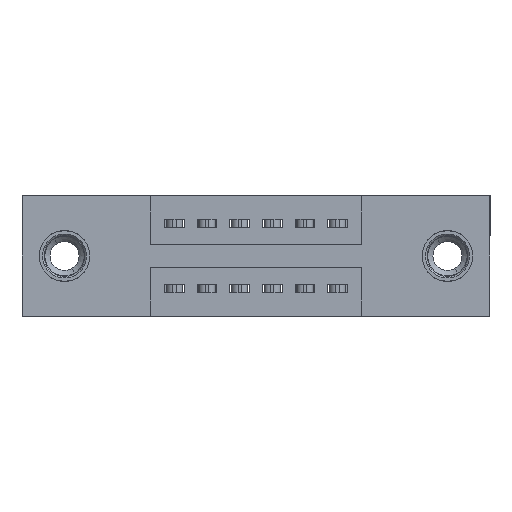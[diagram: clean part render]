
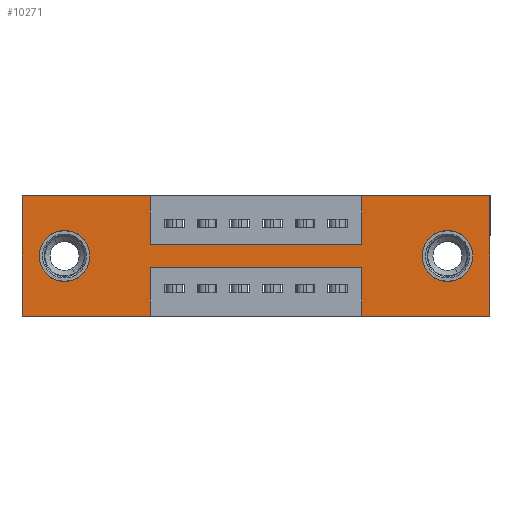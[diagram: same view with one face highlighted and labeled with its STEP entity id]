
A CAD part, front view. The second image highlights one B-rep face of the part: STEP entity #10271.
In plain terms, the highlighted planar face has unit normal (0, -1, 0).
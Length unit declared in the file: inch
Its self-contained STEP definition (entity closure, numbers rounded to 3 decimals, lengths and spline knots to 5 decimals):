
#71 = CARTESIAN_POINT ( 'NONE',  ( 1.305, 0., -0.107 ) ) ;
#195 = CARTESIAN_POINT ( 'NONE',  ( 1.0425, 0., 0. ) ) ;
#309 = FACE_BOUND ( 'NONE', #2899, .T. ) ;
#329 = VERTEX_POINT ( 'NONE', #5077 ) ;
#443 = LINE ( 'NONE', #3938, #9184 ) ;
#509 = VERTEX_POINT ( 'NONE', #8169 ) ;
#593 = VERTEX_POINT ( 'NONE', #8720 ) ;
#978 = CARTESIAN_POINT ( 'NONE',  ( 1.305, 0., -0.263 ) ) ;
#1012 = CARTESIAN_POINT ( 'NONE',  ( 1.435, 0., 0. ) ) ;
#1081 = CARTESIAN_POINT ( 'NONE',  ( 0.13, 0., -0.185 ) ) ;
#1207 = LINE ( 'NONE', #6650, #5820 ) ;
#1309 = VERTEX_POINT ( 'NONE', #8824 ) ;
#1321 = EDGE_CURVE ( 'NONE', #329, #1309, #13550, .T. ) ;
#1327 = VECTOR ( 'NONE', #13985, 39.37008 ) ;
#1766 = EDGE_CURVE ( 'NONE', #7419, #8603, #5643, .T. ) ;
#1823 = DIRECTION ( 'NONE',  ( 1., 0., 0. ) ) ;
#1833 = DIRECTION ( 'NONE',  ( -1., 0., 0. ) ) ;
#1854 = LINE ( 'NONE', #4841, #3917 ) ;
#1885 = CARTESIAN_POINT ( 'NONE',  ( 0., 0., -0.37 ) ) ;
#2115 = VECTOR ( 'NONE', #11081, 39.37008 ) ;
#2276 = VECTOR ( 'NONE', #7738, 39.37008 ) ;
#2292 = ORIENTED_EDGE ( 'NONE', *, *, #6326, .T. ) ;
#2359 = FACE_BOUND ( 'NONE', #3261, .T. ) ;
#2613 = CARTESIAN_POINT ( 'NONE',  ( 0., 0., -0.37 ) ) ;
#2625 = LINE ( 'NONE', #5478, #2115 ) ;
#2825 = ORIENTED_EDGE ( 'NONE', *, *, #12207, .F. ) ;
#2860 = DIRECTION ( 'NONE',  ( 1., 0., 0. ) ) ;
#2899 = EDGE_LOOP ( 'NONE', ( #2292, #7243 ) ) ;
#3005 = DIRECTION ( 'NONE',  ( 0., 1., 0. ) ) ;
#3022 = FACE_OUTER_BOUND ( 'NONE', #5416, .T. ) ;
#3121 = DIRECTION ( 'NONE',  ( 0., 0., -1. ) ) ;
#3175 = VECTOR ( 'NONE', #3121, 39.37008 ) ;
#3261 = EDGE_LOOP ( 'NONE', ( #14013, #10385 ) ) ;
#3292 = CARTESIAN_POINT ( 'NONE',  ( 1.305, 0., -0.185 ) ) ;
#3336 = EDGE_CURVE ( 'NONE', #6189, #5545, #10961, .T. ) ;
#3424 = DIRECTION ( 'NONE',  ( 0., 0., 1. ) ) ;
#3454 = CARTESIAN_POINT ( 'NONE',  ( 0.3925, 0., -0.15 ) ) ;
#3520 = EDGE_CURVE ( 'NONE', #1309, #13283, #1207, .T. ) ;
#3569 = VERTEX_POINT ( 'NONE', #6390 ) ;
#3840 = ORIENTED_EDGE ( 'NONE', *, *, #12914, .F. ) ;
#3897 = CARTESIAN_POINT ( 'NONE',  ( 0.13, 0., -0.263 ) ) ;
#3917 = VECTOR ( 'NONE', #9228, 39.37008 ) ;
#3938 = CARTESIAN_POINT ( 'NONE',  ( 0., 0., 0. ) ) ;
#3956 = VERTEX_POINT ( 'NONE', #12489 ) ;
#3997 = DIRECTION ( 'NONE',  ( 0., 0., -1. ) ) ;
#4083 = VERTEX_POINT ( 'NONE', #3897 ) ;
#4121 = DIRECTION ( 'NONE',  ( 0., 1., 0. ) ) ;
#4261 = ORIENTED_EDGE ( 'NONE', *, *, #3336, .F. ) ;
#4343 = CARTESIAN_POINT ( 'NONE',  ( 1.435, 0., 0. ) ) ;
#4669 = PLANE ( 'NONE',  #13917 ) ;
#4761 = VECTOR ( 'NONE', #6535, 39.37008 ) ;
#4841 = CARTESIAN_POINT ( 'NONE',  ( 0.3925, 0., -0.37 ) ) ;
#4990 = ORIENTED_EDGE ( 'NONE', *, *, #6312, .F. ) ;
#5055 = VECTOR ( 'NONE', #1833, 39.37008 ) ;
#5077 = CARTESIAN_POINT ( 'NONE',  ( 0.3925, 0., -0.15 ) ) ;
#5160 = EDGE_CURVE ( 'NONE', #13283, #6378, #443, .T. ) ;
#5214 = DIRECTION ( 'NONE',  ( 0., 0., 1. ) ) ;
#5416 = EDGE_LOOP ( 'NONE', ( #7513, #14264, #13827, #2825, #13492, #11501, #10953, #7540, #8668, #3840, #4261, #4990 ) ) ;
#5478 = CARTESIAN_POINT ( 'NONE',  ( 0., 0., -0.37 ) ) ;
#5539 = CIRCLE ( 'NONE', #8283, 0.078 ) ;
#5545 = VERTEX_POINT ( 'NONE', #5943 ) ;
#5643 = CIRCLE ( 'NONE', #10445, 0.078 ) ;
#5820 = VECTOR ( 'NONE', #3424, 39.37008 ) ;
#5943 = CARTESIAN_POINT ( 'NONE',  ( 0., 0., 0. ) ) ;
#6156 = AXIS2_PLACEMENT_3D ( 'NONE', #11827, #4121, #5214 ) ;
#6189 = VERTEX_POINT ( 'NONE', #1885 ) ;
#6204 = VERTEX_POINT ( 'NONE', #10633 ) ;
#6243 = CARTESIAN_POINT ( 'NONE',  ( 1.435, 0., -0.37 ) ) ;
#6249 = LINE ( 'NONE', #2613, #6939 ) ;
#6312 = EDGE_CURVE ( 'NONE', #3569, #6189, #2625, .T. ) ;
#6326 = EDGE_CURVE ( 'NONE', #8603, #7419, #5539, .T. ) ;
#6378 = VERTEX_POINT ( 'NONE', #4343 ) ;
#6390 = CARTESIAN_POINT ( 'NONE',  ( 0.3925, 0., -0.37 ) ) ;
#6535 = DIRECTION ( 'NONE',  ( 1., 0., 0. ) ) ;
#6576 = EDGE_CURVE ( 'NONE', #11487, #509, #8087, .T. ) ;
#6650 = CARTESIAN_POINT ( 'NONE',  ( 1.0425, 0., 0. ) ) ;
#6658 = EDGE_CURVE ( 'NONE', #4083, #593, #9472, .T. ) ;
#6665 = DIRECTION ( 'NONE',  ( 0., 0., -1. ) ) ;
#6939 = VECTOR ( 'NONE', #13419, 39.37008 ) ;
#6958 = CIRCLE ( 'NONE', #6156, 0.078 ) ;
#7243 = ORIENTED_EDGE ( 'NONE', *, *, #1766, .T. ) ;
#7271 = LINE ( 'NONE', #13816, #11453 ) ;
#7419 = VERTEX_POINT ( 'NONE', #978 ) ;
#7513 = ORIENTED_EDGE ( 'NONE', *, *, #9551, .F. ) ;
#7540 = ORIENTED_EDGE ( 'NONE', *, *, #1321, .F. ) ;
#7548 = DIRECTION ( 'NONE',  ( 0., 0., 1. ) ) ;
#7596 = DIRECTION ( 'NONE',  ( 0., 1., 0. ) ) ;
#7738 = DIRECTION ( 'NONE',  ( 0., 0., 1. ) ) ;
#8087 = LINE ( 'NONE', #12162, #2276 ) ;
#8169 = CARTESIAN_POINT ( 'NONE',  ( 1.0425, 0., -0.22 ) ) ;
#8283 = AXIS2_PLACEMENT_3D ( 'NONE', #10558, #3005, #11730 ) ;
#8317 = LINE ( 'NONE', #8442, #5055 ) ;
#8442 = CARTESIAN_POINT ( 'NONE',  ( 0.3925, 0., -0.22 ) ) ;
#8519 = DIRECTION ( 'NONE',  ( 0., 0., -1. ) ) ;
#8603 = VERTEX_POINT ( 'NONE', #71 ) ;
#8668 = ORIENTED_EDGE ( 'NONE', *, *, #12662, .F. ) ;
#8690 = CARTESIAN_POINT ( 'NONE',  ( 0.3925, 0., 0. ) ) ;
#8720 = CARTESIAN_POINT ( 'NONE',  ( 0.13, 0., -0.107 ) ) ;
#8824 = CARTESIAN_POINT ( 'NONE',  ( 1.0425, 0., -0.15 ) ) ;
#8852 = VERTEX_POINT ( 'NONE', #6243 ) ;
#9184 = VECTOR ( 'NONE', #1823, 39.37008 ) ;
#9228 = DIRECTION ( 'NONE',  ( 0., 0., -1. ) ) ;
#9286 = DIRECTION ( 'NONE',  ( 0., -1., 0. ) ) ;
#9472 = CIRCLE ( 'NONE', #13996, 0.078 ) ;
#9551 = EDGE_CURVE ( 'NONE', #6204, #3569, #1854, .T. ) ;
#9648 = EDGE_CURVE ( 'NONE', #593, #4083, #6958, .T. ) ;
#9712 = CARTESIAN_POINT ( 'NONE',  ( 0., 0., 0. ) ) ;
#10271 = ADVANCED_FACE ( 'NONE', ( #309, #2359, #3022 ), #4669, .T. ) ;
#10385 = ORIENTED_EDGE ( 'NONE', *, *, #6658, .T. ) ;
#10445 = AXIS2_PLACEMENT_3D ( 'NONE', #3292, #7596, #6665 ) ;
#10558 = CARTESIAN_POINT ( 'NONE',  ( 1.305, 0., -0.185 ) ) ;
#10633 = CARTESIAN_POINT ( 'NONE',  ( 0.3925, 0., -0.22 ) ) ;
#10953 = ORIENTED_EDGE ( 'NONE', *, *, #3520, .F. ) ;
#10961 = LINE ( 'NONE', #9712, #1327 ) ;
#11058 = CARTESIAN_POINT ( 'NONE',  ( 1.0425, 0., -0.37 ) ) ;
#11081 = DIRECTION ( 'NONE',  ( -1., 0., 0. ) ) ;
#11340 = EDGE_CURVE ( 'NONE', #6378, #8852, #12196, .T. ) ;
#11453 = VECTOR ( 'NONE', #2860, 39.37008 ) ;
#11487 = VERTEX_POINT ( 'NONE', #11058 ) ;
#11501 = ORIENTED_EDGE ( 'NONE', *, *, #5160, .F. ) ;
#11669 = CARTESIAN_POINT ( 'NONE',  ( 0., 0., -0.37 ) ) ;
#11730 = DIRECTION ( 'NONE',  ( 0., 0., -1. ) ) ;
#11827 = CARTESIAN_POINT ( 'NONE',  ( 0.13, 0., -0.185 ) ) ;
#12162 = CARTESIAN_POINT ( 'NONE',  ( 1.0425, 0., -0.37 ) ) ;
#12196 = LINE ( 'NONE', #1012, #12545 ) ;
#12207 = EDGE_CURVE ( 'NONE', #8852, #11487, #6249, .T. ) ;
#12489 = CARTESIAN_POINT ( 'NONE',  ( 0.3925, 0., 0. ) ) ;
#12538 = EDGE_CURVE ( 'NONE', #509, #6204, #8317, .T. ) ;
#12545 = VECTOR ( 'NONE', #8519, 39.37008 ) ;
#12662 = EDGE_CURVE ( 'NONE', #3956, #329, #14009, .T. ) ;
#12914 = EDGE_CURVE ( 'NONE', #5545, #3956, #7271, .T. ) ;
#13283 = VERTEX_POINT ( 'NONE', #195 ) ;
#13419 = DIRECTION ( 'NONE',  ( -1., 0., 0. ) ) ;
#13492 = ORIENTED_EDGE ( 'NONE', *, *, #11340, .F. ) ;
#13550 = LINE ( 'NONE', #3454, #4761 ) ;
#13816 = CARTESIAN_POINT ( 'NONE',  ( 0., 0., 0. ) ) ;
#13827 = ORIENTED_EDGE ( 'NONE', *, *, #6576, .F. ) ;
#13917 = AXIS2_PLACEMENT_3D ( 'NONE', #11669, #9286, #3997 ) ;
#13985 = DIRECTION ( 'NONE',  ( 0., 0., 1. ) ) ;
#13996 = AXIS2_PLACEMENT_3D ( 'NONE', #1081, #14164, #7548 ) ;
#14009 = LINE ( 'NONE', #8690, #3175 ) ;
#14013 = ORIENTED_EDGE ( 'NONE', *, *, #9648, .T. ) ;
#14164 = DIRECTION ( 'NONE',  ( 0., 1., 0. ) ) ;
#14264 = ORIENTED_EDGE ( 'NONE', *, *, #12538, .F. ) ;
